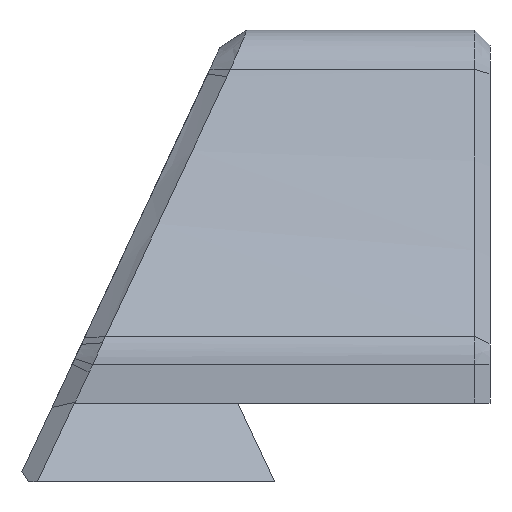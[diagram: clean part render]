
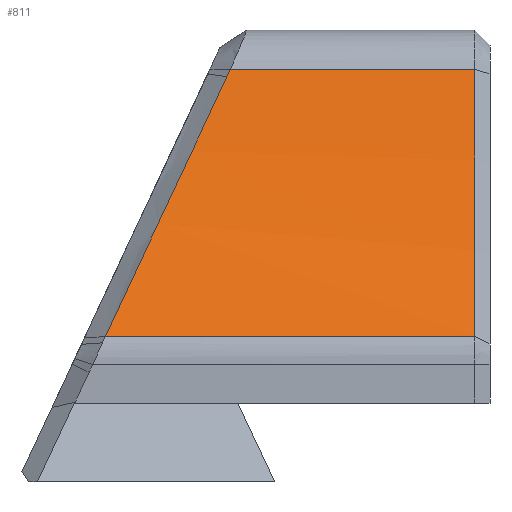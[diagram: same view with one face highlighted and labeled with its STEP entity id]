
A CAD part, left-side view. The second image highlights one B-rep face of the part: STEP entity #811.
In plain terms, the highlighted cylindrical face has radius 37.164 mm (diameter 74.327 mm), a partial arc.
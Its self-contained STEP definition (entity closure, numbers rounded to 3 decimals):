
#72=B_SPLINE_CURVE_WITH_KNOTS('',3,(#1420,#1421,#1422,#1423),
 .UNSPECIFIED.,.F.,.F.,(4,4),(1.058,1.263),
 .UNSPECIFIED.);
#75=B_SPLINE_CURVE_WITH_KNOTS('',3,(#1512,#1513,#1514,#1515),
 .UNSPECIFIED.,.F.,.F.,(4,4),(-1.263,-1.133),
 .UNSPECIFIED.);
#81=CYLINDRICAL_SURFACE('',#877,37.164);
#144=LINE('',#1614,#216);
#145=LINE('',#1616,#217);
#216=VECTOR('',#1036,10.);
#217=VECTOR('',#1039,10.);
#273=FACE_OUTER_BOUND('',#322,.T.);
#322=EDGE_LOOP('',(#729,#730,#731,#732,#733));
#346=CIRCLE('',#861,37.164);
#373=VERTEX_POINT('',#1148);
#374=VERTEX_POINT('',#1152);
#411=VERTEX_POINT('',#1417);
#412=VERTEX_POINT('',#1419);
#413=VERTEX_POINT('',#1465);
#457=EDGE_CURVE('',#373,#374,#346,.T.);
#506=EDGE_CURVE('',#411,#412,#72,.T.);
#514=EDGE_CURVE('',#412,#413,#75,.T.);
#526=EDGE_CURVE('',#413,#373,#144,.T.);
#527=EDGE_CURVE('',#374,#411,#145,.T.);
#729=ORIENTED_EDGE('',*,*,#457,.F.);
#730=ORIENTED_EDGE('',*,*,#526,.F.);
#731=ORIENTED_EDGE('',*,*,#514,.F.);
#732=ORIENTED_EDGE('',*,*,#506,.F.);
#733=ORIENTED_EDGE('',*,*,#527,.F.);
#811=ADVANCED_FACE('',(#273),#81,.F.);
#861=AXIS2_PLACEMENT_3D('',#1154,#962,#963);
#877=AXIS2_PLACEMENT_3D('',#1615,#1037,#1038);
#962=DIRECTION('center_axis',(0.,1.,0.));
#963=DIRECTION('ref_axis',(0.864,0.,-0.504));
#1036=DIRECTION('',(0.,-1.,0.));
#1037=DIRECTION('center_axis',(0.,1.,0.));
#1038=DIRECTION('ref_axis',(0.864,0.,-0.504));
#1039=DIRECTION('',(0.,1.,0.));
#1148=CARTESIAN_POINT('',(-6.185,-5.78,10.995));
#1152=CARTESIAN_POINT('',(-9.304,-5.78,3.875));
#1154=CARTESIAN_POINT('Origin',(-41.599,-5.78,22.262));
#1417=CARTESIAN_POINT('',(-9.304,4.071,3.875));
#1419=CARTESIAN_POINT('',(-6.247,0.83,10.802));
#1420=CARTESIAN_POINT('Ctrl Pts',(-9.304,4.071,3.875));
#1421=CARTESIAN_POINT('Ctrl Pts',(-8.053,3.043,6.071));
#1422=CARTESIAN_POINT('Ctrl Pts',(-7.027,1.955,8.396));
#1423=CARTESIAN_POINT('Ctrl Pts',(-6.247,0.83,10.802));
#1465=CARTESIAN_POINT('',(-6.185,0.741,10.995));
#1512=CARTESIAN_POINT('Ctrl Pts',(-6.247,0.83,10.802));
#1513=CARTESIAN_POINT('Ctrl Pts',(-6.226,0.8,10.866));
#1514=CARTESIAN_POINT('Ctrl Pts',(-6.206,0.77,10.93));
#1515=CARTESIAN_POINT('Ctrl Pts',(-6.185,0.741,10.995));
#1614=CARTESIAN_POINT('',(-6.185,-5.38,10.995));
#1615=CARTESIAN_POINT('Origin',(-41.599,-5.38,22.262));
#1616=CARTESIAN_POINT('',(-9.304,-5.38,3.875));
